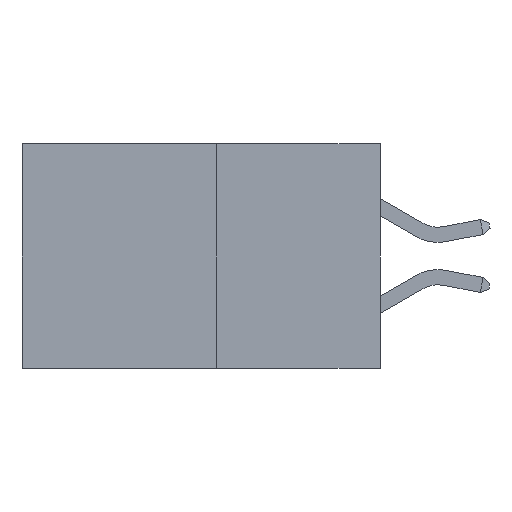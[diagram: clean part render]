
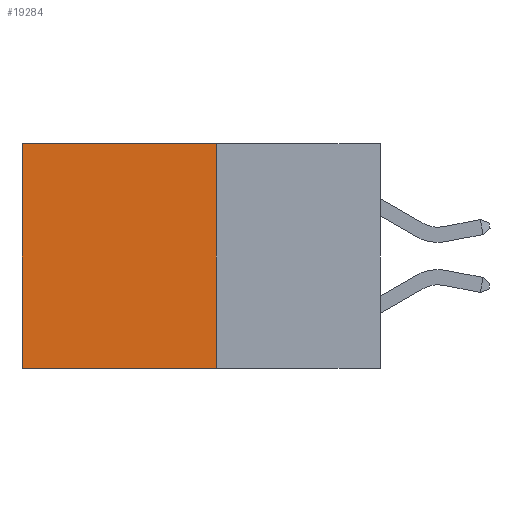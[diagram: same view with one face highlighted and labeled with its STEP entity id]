
A CAD part, left-side view. The second image highlights one B-rep face of the part: STEP entity #19284.
In plain terms, the highlighted planar face has unit normal (-1, 0, 0).
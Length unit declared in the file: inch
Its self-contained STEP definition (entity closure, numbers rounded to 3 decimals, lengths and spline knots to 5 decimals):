
#344 = CARTESIAN_POINT ( 'NONE',  ( 0.277, 0.27, 0. ) ) ;
#1036 = VECTOR ( 'NONE', #15799, 39.37008 ) ;
#1298 = VECTOR ( 'NONE', #4020, 39.37008 ) ;
#2122 = EDGE_CURVE ( 'NONE', #20933, #10246, #22772, .T. ) ;
#4020 = DIRECTION ( 'NONE',  ( 0., 0., -1. ) ) ;
#4967 = EDGE_LOOP ( 'NONE', ( #24174, #17400, #15138, #14862 ) ) ;
#5009 = CARTESIAN_POINT ( 'NONE',  ( 0.277, 0.59, 0. ) ) ;
#5628 = LINE ( 'NONE', #344, #1036 ) ;
#7042 = VECTOR ( 'NONE', #8856, 39.37008 ) ;
#7088 = CARTESIAN_POINT ( 'NONE',  ( 0.277, 0.27, -0.37 ) ) ;
#8856 = DIRECTION ( 'NONE',  ( 0., 0., -1. ) ) ;
#10246 = VERTEX_POINT ( 'NONE', #14123 ) ;
#10578 = FACE_OUTER_BOUND ( 'NONE', #4967, .T. ) ;
#10998 = CARTESIAN_POINT ( 'NONE',  ( 0.277, 0.27, -0.37 ) ) ;
#11148 = VECTOR ( 'NONE', #12918, 39.37008 ) ;
#11237 = DIRECTION ( 'NONE',  ( 0., 0., -1. ) ) ;
#11532 = EDGE_CURVE ( 'NONE', #17638, #20933, #5628, .T. ) ;
#11869 = VERTEX_POINT ( 'NONE', #7088 ) ;
#12918 = DIRECTION ( 'NONE',  ( 0., 1., 0. ) ) ;
#14123 = CARTESIAN_POINT ( 'NONE',  ( 0.277, 0.59, -0.37 ) ) ;
#14862 = ORIENTED_EDGE ( 'NONE', *, *, #11532, .T. ) ;
#15138 = ORIENTED_EDGE ( 'NONE', *, *, #24445, .F. ) ;
#15630 = CARTESIAN_POINT ( 'NONE',  ( 0.277, 0.59, -0.37 ) ) ;
#15799 = DIRECTION ( 'NONE',  ( 0., 1., 0. ) ) ;
#16223 = LINE ( 'NONE', #10998, #11148 ) ;
#16301 = CARTESIAN_POINT ( 'NONE',  ( 0.277, 0.27, 0. ) ) ;
#17400 = ORIENTED_EDGE ( 'NONE', *, *, #21666, .F. ) ;
#17638 = VERTEX_POINT ( 'NONE', #16301 ) ;
#19284 = ADVANCED_FACE ( 'NONE', ( #10578 ), #24299, .F. ) ;
#19305 = CARTESIAN_POINT ( 'NONE',  ( 0.277, 0.27, -0.37 ) ) ;
#20672 = CARTESIAN_POINT ( 'NONE',  ( 0.277, 0.27, -0.37 ) ) ;
#20933 = VERTEX_POINT ( 'NONE', #5009 ) ;
#21354 = AXIS2_PLACEMENT_3D ( 'NONE', #20672, #22537, #11237 ) ;
#21666 = EDGE_CURVE ( 'NONE', #11869, #10246, #16223, .T. ) ;
#21691 = LINE ( 'NONE', #19305, #1298 ) ;
#22537 = DIRECTION ( 'NONE',  ( 1., 0., 0. ) ) ;
#22772 = LINE ( 'NONE', #15630, #7042 ) ;
#24174 = ORIENTED_EDGE ( 'NONE', *, *, #2122, .T. ) ;
#24299 = PLANE ( 'NONE',  #21354 ) ;
#24445 = EDGE_CURVE ( 'NONE', #17638, #11869, #21691, .T. ) ;
